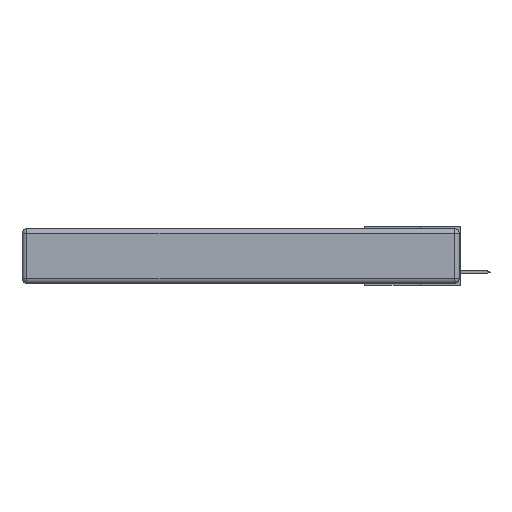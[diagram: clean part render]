
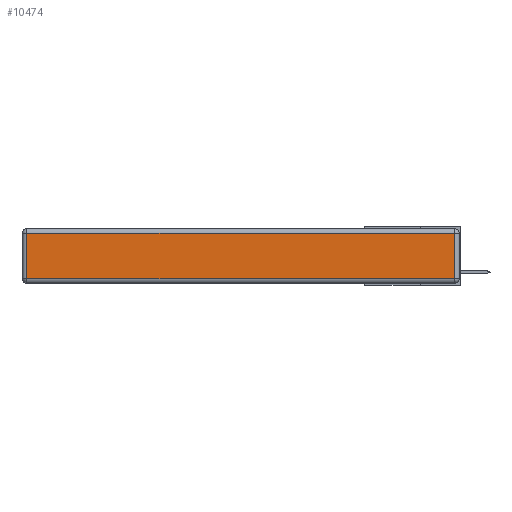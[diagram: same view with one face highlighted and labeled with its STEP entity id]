
A CAD part, left-side view. The second image highlights one B-rep face of the part: STEP entity #10474.
In plain terms, the highlighted planar face has unit normal (-1, 0, 0).
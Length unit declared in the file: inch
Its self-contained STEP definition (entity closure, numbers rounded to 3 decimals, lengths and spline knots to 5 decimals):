
#1676 = ORIENTED_EDGE ( 'NONE', *, *, #3837, .T. ) ;
#1699 = DIRECTION ( 'NONE',  ( 0., -1., 0. ) ) ;
#2944 = CARTESIAN_POINT ( 'NONE',  ( 0., 0.03, -0.343 ) ) ;
#3837 = EDGE_CURVE ( 'NONE', #5836, #13328, #13196, .T. ) ;
#3869 = CARTESIAN_POINT ( 'NONE',  ( 0., 0., -0.313 ) ) ;
#5014 = EDGE_CURVE ( 'NONE', #6961, #5836, #5368, .T. ) ;
#5163 = DIRECTION ( 'NONE',  ( 0., 0., -1. ) ) ;
#5368 = LINE ( 'NONE', #13381, #6666 ) ;
#5836 = VERTEX_POINT ( 'NONE', #12103 ) ;
#6010 = LINE ( 'NONE', #9585, #12348 ) ;
#6287 = DIRECTION ( 'NONE',  ( 0., 1., 0. ) ) ;
#6666 = VECTOR ( 'NONE', #5163, 39.37008 ) ;
#6961 = VERTEX_POINT ( 'NONE', #7710 ) ;
#6999 = LINE ( 'NONE', #2944, #10800 ) ;
#7033 = VECTOR ( 'NONE', #1699, 39.37008 ) ;
#7046 = ORIENTED_EDGE ( 'NONE', *, *, #5014, .T. ) ;
#7059 = FACE_OUTER_BOUND ( 'NONE', #14903, .T. ) ;
#7710 = CARTESIAN_POINT ( 'NONE',  ( 0., 2.72, -0.03 ) ) ;
#7943 = DIRECTION ( 'NONE',  ( -1., 0., 0. ) ) ;
#8514 = AXIS2_PLACEMENT_3D ( 'NONE', #14913, #7943, #13803 ) ;
#9585 = CARTESIAN_POINT ( 'NONE',  ( 0., 2.75, -0.03 ) ) ;
#10090 = DIRECTION ( 'NONE',  ( 0., 0., 1. ) ) ;
#10474 = ADVANCED_FACE ( 'NONE', ( #7059 ), #11362, .T. ) ;
#10800 = VECTOR ( 'NONE', #10090, 39.37008 ) ;
#11362 = PLANE ( 'NONE',  #8514 ) ;
#12103 = CARTESIAN_POINT ( 'NONE',  ( 0., 2.72, -0.313 ) ) ;
#12197 = EDGE_CURVE ( 'NONE', #13328, #15033, #6999, .T. ) ;
#12348 = VECTOR ( 'NONE', #6287, 39.37008 ) ;
#13006 = CARTESIAN_POINT ( 'NONE',  ( 0., 0.03, -0.313 ) ) ;
#13196 = LINE ( 'NONE', #3869, #7033 ) ;
#13328 = VERTEX_POINT ( 'NONE', #13006 ) ;
#13381 = CARTESIAN_POINT ( 'NONE',  ( 0., 2.72, -0.343 ) ) ;
#13622 = ORIENTED_EDGE ( 'NONE', *, *, #12197, .T. ) ;
#13803 = DIRECTION ( 'NONE',  ( 0., 0., 1. ) ) ;
#14053 = EDGE_CURVE ( 'NONE', #15033, #6961, #6010, .T. ) ;
#14903 = EDGE_LOOP ( 'NONE', ( #1676, #13622, #14948, #7046 ) ) ;
#14913 = CARTESIAN_POINT ( 'NONE',  ( 0., 0., -0.343 ) ) ;
#14948 = ORIENTED_EDGE ( 'NONE', *, *, #14053, .T. ) ;
#15012 = CARTESIAN_POINT ( 'NONE',  ( 0., 0.03, -0.03 ) ) ;
#15033 = VERTEX_POINT ( 'NONE', #15012 ) ;
